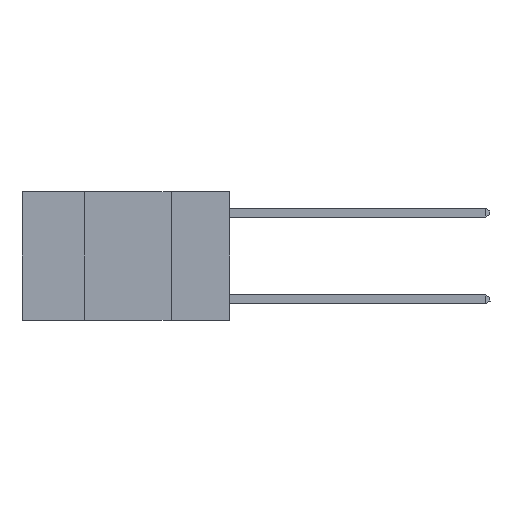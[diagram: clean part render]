
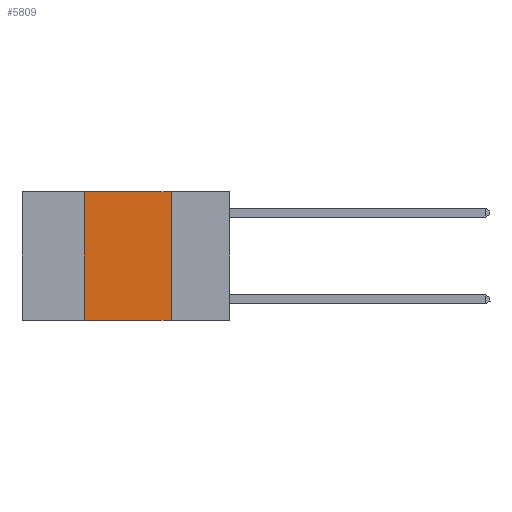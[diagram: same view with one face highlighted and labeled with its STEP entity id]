
A CAD part, left-side view. The second image highlights one B-rep face of the part: STEP entity #5809.
In plain terms, the highlighted planar face has unit normal (-1, 0, 0).
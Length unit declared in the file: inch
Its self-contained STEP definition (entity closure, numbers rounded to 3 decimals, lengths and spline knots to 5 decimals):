
#403 = EDGE_CURVE ( 'NONE', #9029, #3074, #8145, .T. ) ;
#574 = ORIENTED_EDGE ( 'NONE', *, *, #5660, .F. ) ;
#1537 = EDGE_LOOP ( 'NONE', ( #574, #4201, #7439, #11015 ) ) ;
#1558 = EDGE_CURVE ( 'NONE', #9029, #3236, #8303, .T. ) ;
#1604 = CARTESIAN_POINT ( 'NONE',  ( 0., 0.42, 0. ) ) ;
#1799 = VECTOR ( 'NONE', #8255, 39.37008 ) ;
#2198 = CARTESIAN_POINT ( 'NONE',  ( 0., 0.6, 0. ) ) ;
#2557 = CARTESIAN_POINT ( 'NONE',  ( 0., 0.17, -0.37 ) ) ;
#2571 = CARTESIAN_POINT ( 'NONE',  ( 0., 0.6, -0.37 ) ) ;
#3074 = VERTEX_POINT ( 'NONE', #2557 ) ;
#3236 = VERTEX_POINT ( 'NONE', #1604 ) ;
#4028 = LINE ( 'NONE', #8090, #7260 ) ;
#4201 = ORIENTED_EDGE ( 'NONE', *, *, #10752, .F. ) ;
#4709 = VECTOR ( 'NONE', #14222, 39.37008 ) ;
#4766 = CARTESIAN_POINT ( 'NONE',  ( 0., 0.17, 0. ) ) ;
#5660 = EDGE_CURVE ( 'NONE', #6391, #3074, #4028, .T. ) ;
#5809 = ADVANCED_FACE ( 'NONE', ( #14633 ), #14376, .F. ) ;
#6391 = VERTEX_POINT ( 'NONE', #4766 ) ;
#7140 = DIRECTION ( 'NONE',  ( 1., 0., 0. ) ) ;
#7260 = VECTOR ( 'NONE', #9265, 39.37008 ) ;
#7439 = ORIENTED_EDGE ( 'NONE', *, *, #1558, .F. ) ;
#8090 = CARTESIAN_POINT ( 'NONE',  ( 0., 0.17, 0. ) ) ;
#8145 = LINE ( 'NONE', #2571, #14953 ) ;
#8255 = DIRECTION ( 'NONE',  ( 0., -1., 0. ) ) ;
#8303 = LINE ( 'NONE', #13008, #4709 ) ;
#9029 = VERTEX_POINT ( 'NONE', #13219 ) ;
#9265 = DIRECTION ( 'NONE',  ( 0., 0., -1. ) ) ;
#10715 = CARTESIAN_POINT ( 'NONE',  ( 0., 0.6, 0. ) ) ;
#10752 = EDGE_CURVE ( 'NONE', #3236, #6391, #14700, .T. ) ;
#11015 = ORIENTED_EDGE ( 'NONE', *, *, #403, .T. ) ;
#11060 = DIRECTION ( 'NONE',  ( 0., -1., 0. ) ) ;
#11177 = AXIS2_PLACEMENT_3D ( 'NONE', #10715, #7140, #15574 ) ;
#13008 = CARTESIAN_POINT ( 'NONE',  ( 0., 0.42, 0. ) ) ;
#13219 = CARTESIAN_POINT ( 'NONE',  ( 0., 0.42, -0.37 ) ) ;
#14222 = DIRECTION ( 'NONE',  ( 0., 0., 1. ) ) ;
#14376 = PLANE ( 'NONE',  #11177 ) ;
#14633 = FACE_OUTER_BOUND ( 'NONE', #1537, .T. ) ;
#14700 = LINE ( 'NONE', #2198, #1799 ) ;
#14953 = VECTOR ( 'NONE', #11060, 39.37008 ) ;
#15574 = DIRECTION ( 'NONE',  ( 0., 0., -1. ) ) ;
